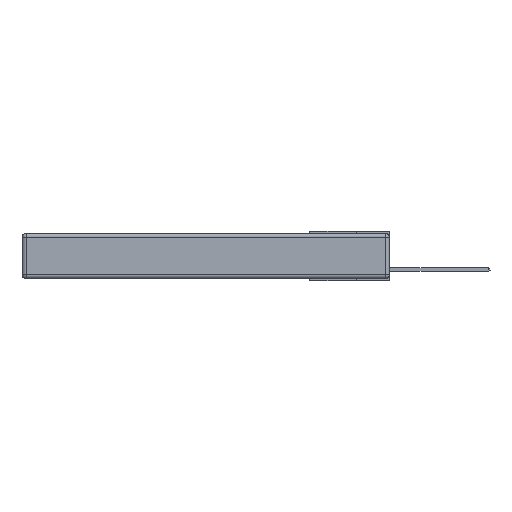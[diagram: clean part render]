
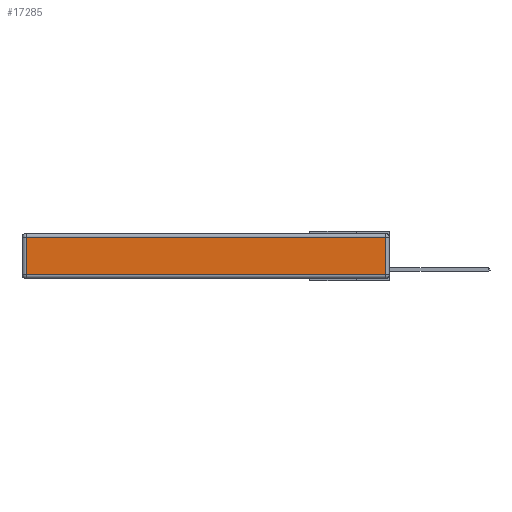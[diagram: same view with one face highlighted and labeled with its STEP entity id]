
A CAD part, left-side view. The second image highlights one B-rep face of the part: STEP entity #17285.
In plain terms, the highlighted planar face has unit normal (-1, 0, 0).
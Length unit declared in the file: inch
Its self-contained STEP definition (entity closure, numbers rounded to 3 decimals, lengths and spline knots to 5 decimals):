
#160 = EDGE_CURVE ( 'NONE', #17102, #9963, #12761, .T. ) ;
#563 = ORIENTED_EDGE ( 'NONE', *, *, #11750, .T. ) ;
#635 = ORIENTED_EDGE ( 'NONE', *, *, #160, .T. ) ;
#1127 = ORIENTED_EDGE ( 'NONE', *, *, #15911, .T. ) ;
#1302 = DIRECTION ( 'NONE',  ( 0., -1., 0. ) ) ;
#1598 = DIRECTION ( 'NONE',  ( 0., 0., -1. ) ) ;
#2141 = CARTESIAN_POINT ( 'NONE',  ( 0., 0.03, -0.03 ) ) ;
#2896 = EDGE_LOOP ( 'NONE', ( #635, #1127, #4780, #563 ) ) ;
#3009 = CARTESIAN_POINT ( 'NONE',  ( 0., 2.72, -0.03 ) ) ;
#3260 = VECTOR ( 'NONE', #1598, 39.37008 ) ;
#3666 = CARTESIAN_POINT ( 'NONE',  ( 0., 2.75, -0.03 ) ) ;
#4680 = CARTESIAN_POINT ( 'NONE',  ( 0., 0., -0.313 ) ) ;
#4780 = ORIENTED_EDGE ( 'NONE', *, *, #16248, .T. ) ;
#5918 = LINE ( 'NONE', #3666, #17672 ) ;
#7225 = DIRECTION ( 'NONE',  ( 0., 0., 1. ) ) ;
#7981 = DIRECTION ( 'NONE',  ( 0., 1., 0. ) ) ;
#9963 = VERTEX_POINT ( 'NONE', #14563 ) ;
#10351 = CARTESIAN_POINT ( 'NONE',  ( 0., 0.03, -0.343 ) ) ;
#10967 = AXIS2_PLACEMENT_3D ( 'NONE', #19519, #14797, #7225 ) ;
#11277 = PLANE ( 'NONE',  #10967 ) ;
#11611 = LINE ( 'NONE', #18679, #3260 ) ;
#11750 = EDGE_CURVE ( 'NONE', #14205, #17102, #11611, .T. ) ;
#11858 = VERTEX_POINT ( 'NONE', #2141 ) ;
#11900 = DIRECTION ( 'NONE',  ( 0., 0., 1. ) ) ;
#12761 = LINE ( 'NONE', #4680, #19495 ) ;
#13620 = VECTOR ( 'NONE', #11900, 39.37008 ) ;
#14205 = VERTEX_POINT ( 'NONE', #3009 ) ;
#14563 = CARTESIAN_POINT ( 'NONE',  ( 0., 0.03, -0.313 ) ) ;
#14797 = DIRECTION ( 'NONE',  ( -1., 0., 0. ) ) ;
#15676 = CARTESIAN_POINT ( 'NONE',  ( 0., 2.72, -0.313 ) ) ;
#15911 = EDGE_CURVE ( 'NONE', #9963, #11858, #17691, .T. ) ;
#16248 = EDGE_CURVE ( 'NONE', #11858, #14205, #5918, .T. ) ;
#17102 = VERTEX_POINT ( 'NONE', #15676 ) ;
#17285 = ADVANCED_FACE ( 'NONE', ( #17401 ), #11277, .T. ) ;
#17401 = FACE_OUTER_BOUND ( 'NONE', #2896, .T. ) ;
#17672 = VECTOR ( 'NONE', #7981, 39.37008 ) ;
#17691 = LINE ( 'NONE', #10351, #13620 ) ;
#18679 = CARTESIAN_POINT ( 'NONE',  ( 0., 2.72, -0.343 ) ) ;
#19495 = VECTOR ( 'NONE', #1302, 39.37008 ) ;
#19519 = CARTESIAN_POINT ( 'NONE',  ( 0., 0., -0.343 ) ) ;
